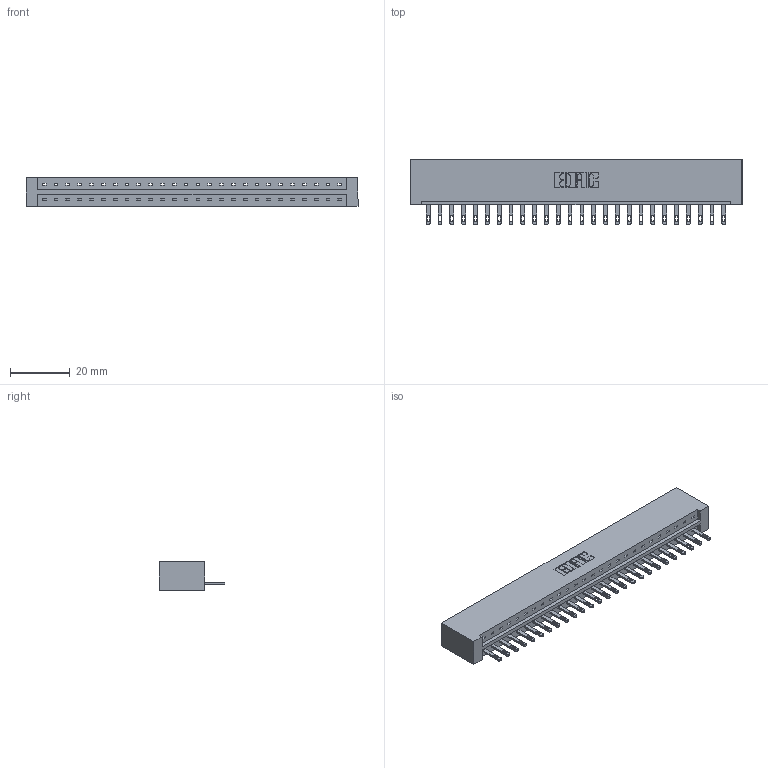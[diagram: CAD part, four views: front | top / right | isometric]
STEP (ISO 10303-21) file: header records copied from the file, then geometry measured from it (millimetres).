
FILE_DESCRIPTION (( 'STEP AP203' ), '1' );
FILE_NAME ('333-026-500-101.STEP', '2018-08-02T12:22:15', ( '' ), ( '' ), 'SwSTEP 2.0', 'SolidWorks 2016', '' );
FILE_SCHEMA (( 'CONFIG_CONTROL_DESIGN' ));
Length unit declared in the file: inch
Products named in the file (3): 333 Part_Lugless; 345-292-001_345-293-100; 333-026-500-101
Assembly tree (27 placements, depth 2):
  333-026-500-101
    333 Part_Lugless
    345-292-001_345-293-100  x26
Bounding box: 111.28 x 21.85 x 9.4 mm (x, y, z)
Volume: 11688.9 mm3; surface area: 12562.1 mm2
Topology: 27 solids, 27 shells, 1510 faces, 4655 edges, 3102 vertices
Faces by surface type: plane 1002, cylinder 508
Entity records: 17617 total; most frequent: CARTESIAN_POINT 3048, ORIENTED_EDGE 3010, DIRECTION 2597, EDGE_CURVE 1505, VECTOR 1381, LINE 1381, VERTEX_POINT 1002, AXIS2_PLACEMENT_3D 608
